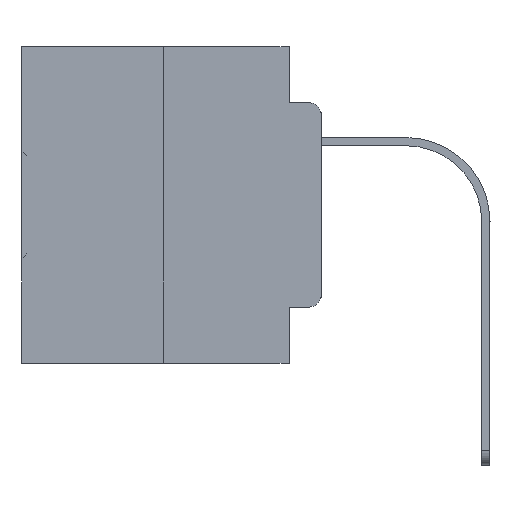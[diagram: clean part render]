
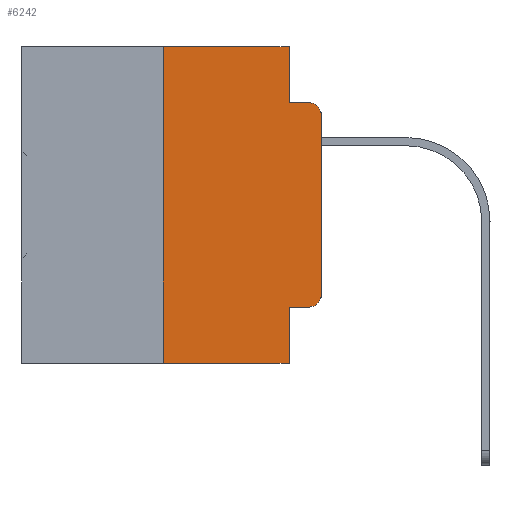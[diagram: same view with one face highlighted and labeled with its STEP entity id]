
A CAD part, left-side view. The second image highlights one B-rep face of the part: STEP entity #6242.
In plain terms, the highlighted planar face has unit normal (-1, 0, 0).
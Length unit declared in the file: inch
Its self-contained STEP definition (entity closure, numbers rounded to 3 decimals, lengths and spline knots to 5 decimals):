
#682 = VERTEX_POINT ( 'NONE', #5932 ) ;
#1615 = VERTEX_POINT ( 'NONE', #27064 ) ;
#1712 = CARTESIAN_POINT ( 'NONE',  ( 0., 0.02, -0.1085 ) ) ;
#2533 = CARTESIAN_POINT ( 'NONE',  ( 0., 0.051, 0. ) ) ;
#2696 = AXIS2_PLACEMENT_3D ( 'NONE', #5108, #24052, #26328 ) ;
#3794 = DIRECTION ( 'NONE',  ( 0., 0., -1. ) ) ;
#4434 = ORIENTED_EDGE ( 'NONE', *, *, #29976, .T. ) ;
#4543 = EDGE_CURVE ( 'NONE', #9734, #17065, #12925, .T. ) ;
#5108 = CARTESIAN_POINT ( 'NONE',  ( 0., 0.02, -0.3915 ) ) ;
#5214 = CARTESIAN_POINT ( 'NONE',  ( 0., 0.25, 0. ) ) ;
#5356 = CIRCLE ( 'NONE', #16491, 0.02 ) ;
#5522 = VERTEX_POINT ( 'NONE', #13659 ) ;
#5585 = AXIS2_PLACEMENT_3D ( 'NONE', #15863, #31125, #28536 ) ;
#5932 = CARTESIAN_POINT ( 'NONE',  ( 0., 0., -0.1085 ) ) ;
#6150 = CARTESIAN_POINT ( 'NONE',  ( 0., 0.473, 0. ) ) ;
#6242 = ADVANCED_FACE ( 'NONE', ( #23638 ), #29050, .F. ) ;
#7254 = CARTESIAN_POINT ( 'NONE',  ( 0., 0., -0.3915 ) ) ;
#7579 = VECTOR ( 'NONE', #13317, 39.37008 ) ;
#8207 = DIRECTION ( 'NONE',  ( 0., 0., -1. ) ) ;
#9098 = ORIENTED_EDGE ( 'NONE', *, *, #15589, .F. ) ;
#9209 = DIRECTION ( 'NONE',  ( -1., 0., 0. ) ) ;
#9734 = VERTEX_POINT ( 'NONE', #33489 ) ;
#9781 = ORIENTED_EDGE ( 'NONE', *, *, #4543, .T. ) ;
#9851 = EDGE_CURVE ( 'NONE', #1615, #15319, #23578, .T. ) ;
#10275 = LINE ( 'NONE', #19134, #12307 ) ;
#10358 = LINE ( 'NONE', #15261, #23489 ) ;
#10989 = EDGE_CURVE ( 'NONE', #28881, #682, #10358, .T. ) ;
#11312 = DIRECTION ( 'NONE',  ( 0., -1., 0. ) ) ;
#12307 = VECTOR ( 'NONE', #11312, 39.37008 ) ;
#12925 = LINE ( 'NONE', #18649, #28996 ) ;
#13092 = DIRECTION ( 'NONE',  ( 0., -1., 0. ) ) ;
#13104 = CARTESIAN_POINT ( 'NONE',  ( 0., 0.051, -0.5 ) ) ;
#13317 = DIRECTION ( 'NONE',  ( 0., -1., 0. ) ) ;
#13659 = CARTESIAN_POINT ( 'NONE',  ( 0., 0.051, -0.4115 ) ) ;
#14115 = EDGE_CURVE ( 'NONE', #15319, #16407, #18563, .T. ) ;
#14131 = EDGE_LOOP ( 'NONE', ( #28055, #4434, #20313, #34281, #9098, #21373, #9781, #29441, #25734, #20005 ) ) ;
#15261 = CARTESIAN_POINT ( 'NONE',  ( 0., 0., 0. ) ) ;
#15319 = VERTEX_POINT ( 'NONE', #32969 ) ;
#15589 = EDGE_CURVE ( 'NONE', #25059, #1615, #26872, .T. ) ;
#15863 = CARTESIAN_POINT ( 'NONE',  ( 0., 0.473, 0. ) ) ;
#16318 = EDGE_CURVE ( 'NONE', #5522, #26607, #10275, .T. ) ;
#16388 = EDGE_CURVE ( 'NONE', #9734, #25059, #26429, .T. ) ;
#16407 = VERTEX_POINT ( 'NONE', #21224 ) ;
#16452 = CARTESIAN_POINT ( 'NONE',  ( 0., 0.02, -0.4115 ) ) ;
#16491 = AXIS2_PLACEMENT_3D ( 'NONE', #1712, #9209, #3794 ) ;
#17065 = VERTEX_POINT ( 'NONE', #13104 ) ;
#18563 = LINE ( 'NONE', #29160, #7579 ) ;
#18649 = CARTESIAN_POINT ( 'NONE',  ( 0., 0.473, -0.5 ) ) ;
#19134 = CARTESIAN_POINT ( 'NONE',  ( 0., 0.051, -0.4115 ) ) ;
#20005 = ORIENTED_EDGE ( 'NONE', *, *, #33631, .T. ) ;
#20313 = ORIENTED_EDGE ( 'NONE', *, *, #14115, .F. ) ;
#21224 = CARTESIAN_POINT ( 'NONE',  ( 0., 0.02, -0.0885 ) ) ;
#21373 = ORIENTED_EDGE ( 'NONE', *, *, #16388, .F. ) ;
#21504 = VECTOR ( 'NONE', #8207, 39.37008 ) ;
#22279 = VECTOR ( 'NONE', #29215, 39.37008 ) ;
#22676 = CIRCLE ( 'NONE', #2696, 0.02 ) ;
#23489 = VECTOR ( 'NONE', #28260, 39.37008 ) ;
#23578 = LINE ( 'NONE', #2533, #25770 ) ;
#23638 = FACE_OUTER_BOUND ( 'NONE', #14131, .T. ) ;
#23896 = DIRECTION ( 'NONE',  ( 0., 0., -1. ) ) ;
#24052 = DIRECTION ( 'NONE',  ( -1., 0., 0. ) ) ;
#25059 = VERTEX_POINT ( 'NONE', #30409 ) ;
#25734 = ORIENTED_EDGE ( 'NONE', *, *, #16318, .T. ) ;
#25770 = VECTOR ( 'NONE', #23896, 39.37008 ) ;
#26328 = DIRECTION ( 'NONE',  ( 0., 0., -1. ) ) ;
#26429 = LINE ( 'NONE', #5214, #22279 ) ;
#26607 = VERTEX_POINT ( 'NONE', #16452 ) ;
#26872 = LINE ( 'NONE', #6150, #33872 ) ;
#27064 = CARTESIAN_POINT ( 'NONE',  ( 0., 0.051, 0. ) ) ;
#28055 = ORIENTED_EDGE ( 'NONE', *, *, #10989, .T. ) ;
#28260 = DIRECTION ( 'NONE',  ( 0., 0., 1. ) ) ;
#28536 = DIRECTION ( 'NONE',  ( 0., 0., -1. ) ) ;
#28755 = CARTESIAN_POINT ( 'NONE',  ( 0., 0.051, 0. ) ) ;
#28881 = VERTEX_POINT ( 'NONE', #7254 ) ;
#28996 = VECTOR ( 'NONE', #13092, 39.37008 ) ;
#29050 = PLANE ( 'NONE',  #5585 ) ;
#29160 = CARTESIAN_POINT ( 'NONE',  ( 0., 0.051, -0.0885 ) ) ;
#29215 = DIRECTION ( 'NONE',  ( 0., 0., 1. ) ) ;
#29441 = ORIENTED_EDGE ( 'NONE', *, *, #32365, .F. ) ;
#29976 = EDGE_CURVE ( 'NONE', #682, #16407, #5356, .T. ) ;
#30409 = CARTESIAN_POINT ( 'NONE',  ( 0., 0.25, 0. ) ) ;
#31125 = DIRECTION ( 'NONE',  ( 1., 0., 0. ) ) ;
#31882 = LINE ( 'NONE', #28755, #21504 ) ;
#32365 = EDGE_CURVE ( 'NONE', #5522, #17065, #31882, .T. ) ;
#32429 = DIRECTION ( 'NONE',  ( 0., -1., 0. ) ) ;
#32969 = CARTESIAN_POINT ( 'NONE',  ( 0., 0.051, -0.0885 ) ) ;
#33489 = CARTESIAN_POINT ( 'NONE',  ( 0., 0.25, -0.5 ) ) ;
#33631 = EDGE_CURVE ( 'NONE', #26607, #28881, #22676, .T. ) ;
#33872 = VECTOR ( 'NONE', #32429, 39.37008 ) ;
#34281 = ORIENTED_EDGE ( 'NONE', *, *, #9851, .F. ) ;
